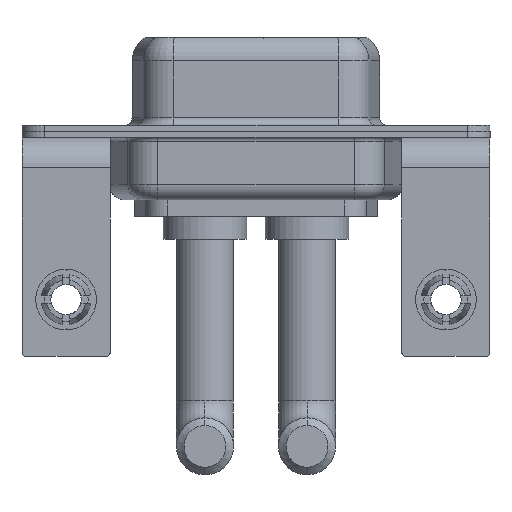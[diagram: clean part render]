
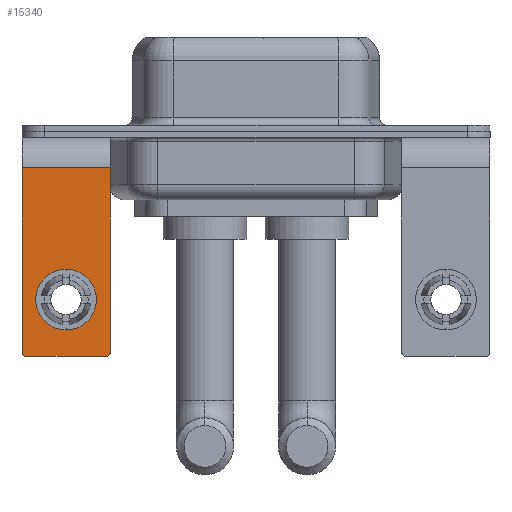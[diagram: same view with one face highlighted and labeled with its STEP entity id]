
A CAD part, front view. The second image highlights one B-rep face of the part: STEP entity #15340.
In plain terms, the highlighted planar face has unit normal (0, -1, 0).
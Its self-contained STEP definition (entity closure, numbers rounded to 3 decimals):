
#85 = CARTESIAN_POINT ( 'NONE',  ( 2.9, -6.25, -2.4 ) ) ;
#281 = DIRECTION ( 'NONE',  ( 0., -1., 0. ) ) ;
#352 = DIRECTION ( 'NONE',  ( 0., 1., 0. ) ) ;
#783 = VERTEX_POINT ( 'NONE', #10291 ) ;
#951 = DIRECTION ( 'NONE',  ( -1., 0., 0. ) ) ;
#981 = CARTESIAN_POINT ( 'NONE',  ( 2.9, -6.25, -14.55 ) ) ;
#1033 = CARTESIAN_POINT ( 'NONE',  ( 0., -6.25, -11.07 ) ) ;
#1108 = VERTEX_POINT ( 'NONE', #1224 ) ;
#1224 = CARTESIAN_POINT ( 'NONE',  ( 0., -6.25, -13.07 ) ) ;
#1235 = ORIENTED_EDGE ( 'NONE', *, *, #4063, .T. ) ;
#1395 = EDGE_CURVE ( 'NONE', #6847, #14407, #2927, .T. ) ;
#1586 = VERTEX_POINT ( 'NONE', #9329 ) ;
#1689 = ORIENTED_EDGE ( 'NONE', *, *, #10881, .T. ) ;
#1873 = AXIS2_PLACEMENT_3D ( 'NONE', #10203, #12520, #13948 ) ;
#2149 = DIRECTION ( 'NONE',  ( 0., 0., -1. ) ) ;
#2927 = LINE ( 'NONE', #15064, #10039 ) ;
#3208 = VECTOR ( 'NONE', #2149, 1000. ) ;
#3342 = CARTESIAN_POINT ( 'NONE',  ( -2.65, -6.25, -14.8 ) ) ;
#3756 = CARTESIAN_POINT ( 'NONE',  ( 2.9, -6.25, -2.4 ) ) ;
#3926 = EDGE_CURVE ( 'NONE', #1586, #10286, #11752, .T. ) ;
#4013 = CARTESIAN_POINT ( 'NONE',  ( 2.65, -6.25, -14.8 ) ) ;
#4063 = EDGE_CURVE ( 'NONE', #1108, #783, #12068, .T. ) ;
#4167 = ORIENTED_EDGE ( 'NONE', *, *, #3926, .T. ) ;
#4578 = CIRCLE ( 'NONE', #12941, 0.25 ) ;
#4579 = EDGE_CURVE ( 'NONE', #10286, #14407, #11781, .T. ) ;
#5702 = ORIENTED_EDGE ( 'NONE', *, *, #14465, .T. ) ;
#5885 = DIRECTION ( 'NONE',  ( 0., 1., 0. ) ) ;
#6033 = DIRECTION ( 'NONE',  ( 0., 0., 1. ) ) ;
#6046 = DIRECTION ( 'NONE',  ( 0., 0., -1. ) ) ;
#6314 = CARTESIAN_POINT ( 'NONE',  ( -2.65, -6.25, -14.55 ) ) ;
#6416 = VECTOR ( 'NONE', #951, 1000. ) ;
#6539 = CARTESIAN_POINT ( 'NONE',  ( 0., -6.25, -11.07 ) ) ;
#6636 = FACE_OUTER_BOUND ( 'NONE', #15501, .T. ) ;
#6847 = VERTEX_POINT ( 'NONE', #4013 ) ;
#6908 = CARTESIAN_POINT ( 'NONE',  ( 2.9, -6.25, -2.4 ) ) ;
#7659 = ORIENTED_EDGE ( 'NONE', *, *, #1395, .F. ) ;
#7982 = AXIS2_PLACEMENT_3D ( 'NONE', #6314, #8926, #11147 ) ;
#8171 = LINE ( 'NONE', #6908, #6416 ) ;
#8487 = VERTEX_POINT ( 'NONE', #85 ) ;
#8926 = DIRECTION ( 'NONE',  ( 0., -1., 0. ) ) ;
#9122 = EDGE_CURVE ( 'NONE', #6847, #12476, #4578, .T. ) ;
#9271 = AXIS2_PLACEMENT_3D ( 'NONE', #1033, #5885, #6033 ) ;
#9329 = CARTESIAN_POINT ( 'NONE',  ( -2.9, -6.25, -2.4 ) ) ;
#9870 = DIRECTION ( 'NONE',  ( 0., 0., 1. ) ) ;
#10004 = LINE ( 'NONE', #3756, #15542 ) ;
#10039 = VECTOR ( 'NONE', #12841, 1000. ) ;
#10190 = AXIS2_PLACEMENT_3D ( 'NONE', #6539, #352, #9870 ) ;
#10203 = CARTESIAN_POINT ( 'NONE',  ( 2.9, -6.25, -2.4 ) ) ;
#10286 = VERTEX_POINT ( 'NONE', #11081 ) ;
#10291 = CARTESIAN_POINT ( 'NONE',  ( 0., -6.25, -9.07 ) ) ;
#10881 = EDGE_CURVE ( 'NONE', #783, #1108, #15013, .T. ) ;
#11081 = CARTESIAN_POINT ( 'NONE',  ( -2.9, -6.25, -14.55 ) ) ;
#11147 = DIRECTION ( 'NONE',  ( 0., 0., 1. ) ) ;
#11154 = CARTESIAN_POINT ( 'NONE',  ( 2.65, -6.25, -14.55 ) ) ;
#11312 = DIRECTION ( 'NONE',  ( 0., 0., 1. ) ) ;
#11469 = PLANE ( 'NONE',  #1873 ) ;
#11752 = LINE ( 'NONE', #14218, #3208 ) ;
#11781 = CIRCLE ( 'NONE', #7982, 0.25 ) ;
#12068 = CIRCLE ( 'NONE', #9271, 2. ) ;
#12396 = ORIENTED_EDGE ( 'NONE', *, *, #14067, .F. ) ;
#12476 = VERTEX_POINT ( 'NONE', #981 ) ;
#12520 = DIRECTION ( 'NONE',  ( 0., 1., 0. ) ) ;
#12635 = EDGE_LOOP ( 'NONE', ( #1235, #1689 ) ) ;
#12841 = DIRECTION ( 'NONE',  ( -1., 0., 0. ) ) ;
#12941 = AXIS2_PLACEMENT_3D ( 'NONE', #11154, #281, #11312 ) ;
#13635 = FACE_BOUND ( 'NONE', #12635, .T. ) ;
#13817 = ORIENTED_EDGE ( 'NONE', *, *, #9122, .T. ) ;
#13948 = DIRECTION ( 'NONE',  ( 0., 0., 1. ) ) ;
#14067 = EDGE_CURVE ( 'NONE', #8487, #12476, #10004, .T. ) ;
#14218 = CARTESIAN_POINT ( 'NONE',  ( -2.9, -6.25, -2.4 ) ) ;
#14407 = VERTEX_POINT ( 'NONE', #3342 ) ;
#14465 = EDGE_CURVE ( 'NONE', #8487, #1586, #8171, .T. ) ;
#15013 = CIRCLE ( 'NONE', #10190, 2. ) ;
#15064 = CARTESIAN_POINT ( 'NONE',  ( 2.9, -6.25, -14.8 ) ) ;
#15325 = ORIENTED_EDGE ( 'NONE', *, *, #4579, .T. ) ;
#15340 = ADVANCED_FACE ( 'NONE', ( #13635, #6636 ), #11469, .F. ) ;
#15501 = EDGE_LOOP ( 'NONE', ( #4167, #15325, #7659, #13817, #12396, #5702 ) ) ;
#15542 = VECTOR ( 'NONE', #6046, 1000. ) ;
